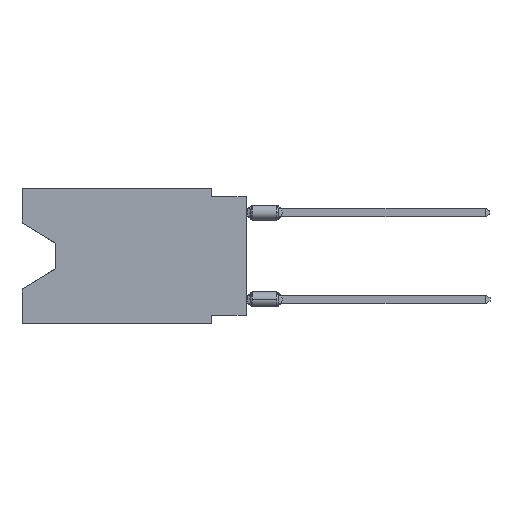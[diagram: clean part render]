
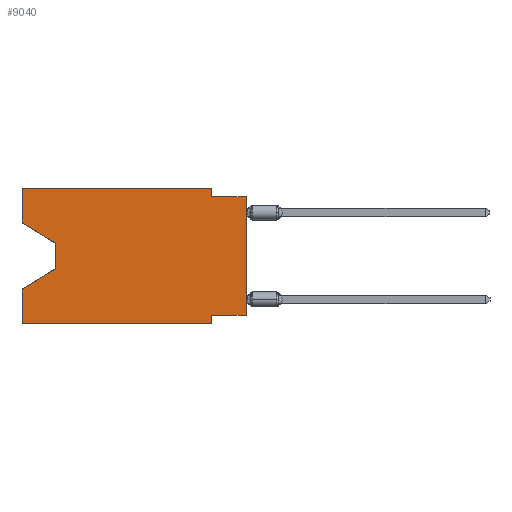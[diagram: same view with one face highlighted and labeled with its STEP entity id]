
A CAD part, left-side view. The second image highlights one B-rep face of the part: STEP entity #9040.
In plain terms, the highlighted planar face has unit normal (-1, 0, 0).
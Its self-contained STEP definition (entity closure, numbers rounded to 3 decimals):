
#80 = DIRECTION ( 'NONE',  ( 0., -1., 0. ) ) ;
#245 = AXIS2_PLACEMENT_3D ( 'NONE', #15525, #9999, #4618 ) ;
#256 = ORIENTED_EDGE ( 'NONE', *, *, #5474, .T. ) ;
#556 = FACE_OUTER_BOUND ( 'NONE', #18193, .T. ) ;
#698 = CARTESIAN_POINT ( 'NONE',  ( 0., 2.54, -9.271 ) ) ;
#1157 = DIRECTION ( 'NONE',  ( 0., -1., 0. ) ) ;
#1538 = CARTESIAN_POINT ( 'NONE',  ( 0., 0., -0.635 ) ) ;
#1731 = LINE ( 'NONE', #10810, #11484 ) ;
#1797 = CARTESIAN_POINT ( 'NONE',  ( 0., 2.54, -0.635 ) ) ;
#1945 = EDGE_CURVE ( 'NONE', #5978, #24084, #8978, .T. ) ;
#2351 = ORIENTED_EDGE ( 'NONE', *, *, #12193, .F. ) ;
#2882 = EDGE_CURVE ( 'NONE', #24084, #3650, #6425, .T. ) ;
#3449 = LINE ( 'NONE', #23976, #18606 ) ;
#3650 = VERTEX_POINT ( 'NONE', #12660 ) ;
#3745 = CARTESIAN_POINT ( 'NONE',  ( 0., 13.97, -5.893 ) ) ;
#3774 = CARTESIAN_POINT ( 'NONE',  ( 0., 16.383, 0. ) ) ;
#3901 = CARTESIAN_POINT ( 'NONE',  ( 0., 2.54, 0. ) ) ;
#4403 = DIRECTION ( 'NONE',  ( 0., 1., 0. ) ) ;
#4476 = CARTESIAN_POINT ( 'NONE',  ( 0., 0., -9.271 ) ) ;
#4618 = DIRECTION ( 'NONE',  ( 0., 0., -1. ) ) ;
#4798 = EDGE_CURVE ( 'NONE', #16609, #13565, #15314, .T. ) ;
#4935 = VECTOR ( 'NONE', #13570, 1000. ) ;
#5211 = ORIENTED_EDGE ( 'NONE', *, *, #5909, .F. ) ;
#5299 = CARTESIAN_POINT ( 'NONE',  ( 0., 16.383, -2.546 ) ) ;
#5438 = LINE ( 'NONE', #10957, #9503 ) ;
#5474 = EDGE_CURVE ( 'NONE', #16609, #7939, #20163, .T. ) ;
#5909 = EDGE_CURVE ( 'NONE', #13565, #7614, #5438, .T. ) ;
#5959 = CARTESIAN_POINT ( 'NONE',  ( 0., 16.383, -9.906 ) ) ;
#5978 = VERTEX_POINT ( 'NONE', #12812 ) ;
#6425 = LINE ( 'NONE', #17586, #4935 ) ;
#6660 = CARTESIAN_POINT ( 'NONE',  ( 0., 16.383, -7.36 ) ) ;
#6675 = VERTEX_POINT ( 'NONE', #6660 ) ;
#6836 = ORIENTED_EDGE ( 'NONE', *, *, #1945, .T. ) ;
#6929 = LINE ( 'NONE', #12574, #13143 ) ;
#7600 = EDGE_CURVE ( 'NONE', #21564, #7614, #11748, .T. ) ;
#7614 = VERTEX_POINT ( 'NONE', #11626 ) ;
#7620 = ORIENTED_EDGE ( 'NONE', *, *, #4798, .F. ) ;
#7939 = VERTEX_POINT ( 'NONE', #1538 ) ;
#8243 = EDGE_CURVE ( 'NONE', #15153, #16522, #3449, .T. ) ;
#8978 = LINE ( 'NONE', #5299, #17822 ) ;
#9040 = ADVANCED_FACE ( 'NONE', ( #556 ), #17600, .F. ) ;
#9503 = VECTOR ( 'NONE', #22307, 1000. ) ;
#9615 = VECTOR ( 'NONE', #19398, 1000. ) ;
#9845 = VECTOR ( 'NONE', #4403, 1000. ) ;
#9945 = CARTESIAN_POINT ( 'NONE',  ( 0., 16.383, 0. ) ) ;
#9999 = DIRECTION ( 'NONE',  ( 1., 0., 0. ) ) ;
#10036 = CARTESIAN_POINT ( 'NONE',  ( 0., 0., -9.271 ) ) ;
#10810 = CARTESIAN_POINT ( 'NONE',  ( 0., 0., -0.635 ) ) ;
#10868 = CARTESIAN_POINT ( 'NONE',  ( 0., 0., 0. ) ) ;
#10957 = CARTESIAN_POINT ( 'NONE',  ( 0., 2.54, -9.906 ) ) ;
#10981 = LINE ( 'NONE', #3745, #11741 ) ;
#11484 = VECTOR ( 'NONE', #18295, 1000. ) ;
#11626 = CARTESIAN_POINT ( 'NONE',  ( 0., 2.54, -9.906 ) ) ;
#11676 = ORIENTED_EDGE ( 'NONE', *, *, #14610, .F. ) ;
#11741 = VECTOR ( 'NONE', #16476, 1000. ) ;
#11748 = LINE ( 'NONE', #5959, #21318 ) ;
#12193 = EDGE_CURVE ( 'NONE', #21564, #6675, #13340, .T. ) ;
#12574 = CARTESIAN_POINT ( 'NONE',  ( 0., 16.383, 0. ) ) ;
#12608 = EDGE_CURVE ( 'NONE', #3650, #6675, #10981, .T. ) ;
#12660 = CARTESIAN_POINT ( 'NONE',  ( 0., 13.97, -5.893 ) ) ;
#12812 = CARTESIAN_POINT ( 'NONE',  ( 0., 16.383, -2.546 ) ) ;
#13143 = VECTOR ( 'NONE', #1157, 1000. ) ;
#13214 = EDGE_CURVE ( 'NONE', #5978, #14923, #17065, .T. ) ;
#13340 = LINE ( 'NONE', #3774, #15624 ) ;
#13565 = VERTEX_POINT ( 'NONE', #698 ) ;
#13570 = DIRECTION ( 'NONE',  ( 0., 0., -1. ) ) ;
#14610 = EDGE_CURVE ( 'NONE', #16522, #7939, #1731, .T. ) ;
#14923 = VERTEX_POINT ( 'NONE', #15796 ) ;
#15153 = VERTEX_POINT ( 'NONE', #3901 ) ;
#15314 = LINE ( 'NONE', #10036, #9845 ) ;
#15525 = CARTESIAN_POINT ( 'NONE',  ( 0., 16.383, 0. ) ) ;
#15624 = VECTOR ( 'NONE', #16995, 1000. ) ;
#15703 = ORIENTED_EDGE ( 'NONE', *, *, #12608, .T. ) ;
#15796 = CARTESIAN_POINT ( 'NONE',  ( 0., 16.383, 0. ) ) ;
#16476 = DIRECTION ( 'NONE',  ( 0., 0.855, -0.519 ) ) ;
#16522 = VERTEX_POINT ( 'NONE', #1797 ) ;
#16609 = VERTEX_POINT ( 'NONE', #4476 ) ;
#16728 = EDGE_CURVE ( 'NONE', #14923, #15153, #6929, .T. ) ;
#16995 = DIRECTION ( 'NONE',  ( 0., 0., 1. ) ) ;
#17065 = LINE ( 'NONE', #9945, #9615 ) ;
#17586 = CARTESIAN_POINT ( 'NONE',  ( 0., 13.97, -4.013 ) ) ;
#17600 = PLANE ( 'NONE',  #245 ) ;
#17822 = VECTOR ( 'NONE', #19896, 1000. ) ;
#18193 = EDGE_LOOP ( 'NONE', ( #6836, #23814, #15703, #2351, #19088, #5211, #7620, #256, #11676, #19006, #20203, #23735 ) ) ;
#18295 = DIRECTION ( 'NONE',  ( 0., -1., 0. ) ) ;
#18606 = VECTOR ( 'NONE', #23620, 1000. ) ;
#19006 = ORIENTED_EDGE ( 'NONE', *, *, #8243, .F. ) ;
#19088 = ORIENTED_EDGE ( 'NONE', *, *, #7600, .T. ) ;
#19398 = DIRECTION ( 'NONE',  ( 0., 0., 1. ) ) ;
#19896 = DIRECTION ( 'NONE',  ( 0., -0.855, -0.519 ) ) ;
#20163 = LINE ( 'NONE', #10868, #21206 ) ;
#20203 = ORIENTED_EDGE ( 'NONE', *, *, #16728, .F. ) ;
#21206 = VECTOR ( 'NONE', #22099, 1000. ) ;
#21318 = VECTOR ( 'NONE', #80, 1000. ) ;
#21564 = VERTEX_POINT ( 'NONE', #22515 ) ;
#21771 = CARTESIAN_POINT ( 'NONE',  ( 0., 13.97, -4.013 ) ) ;
#22099 = DIRECTION ( 'NONE',  ( 0., 0., 1. ) ) ;
#22307 = DIRECTION ( 'NONE',  ( 0., 0., -1. ) ) ;
#22515 = CARTESIAN_POINT ( 'NONE',  ( 0., 16.383, -9.906 ) ) ;
#23620 = DIRECTION ( 'NONE',  ( 0., 0., -1. ) ) ;
#23735 = ORIENTED_EDGE ( 'NONE', *, *, #13214, .F. ) ;
#23814 = ORIENTED_EDGE ( 'NONE', *, *, #2882, .T. ) ;
#23976 = CARTESIAN_POINT ( 'NONE',  ( 0., 2.54, 0. ) ) ;
#24084 = VERTEX_POINT ( 'NONE', #21771 ) ;
